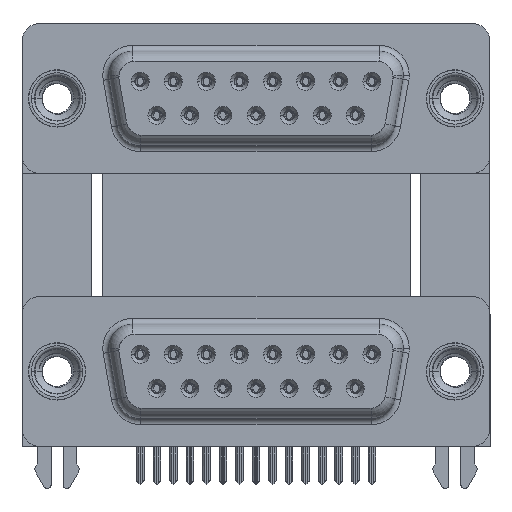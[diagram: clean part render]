
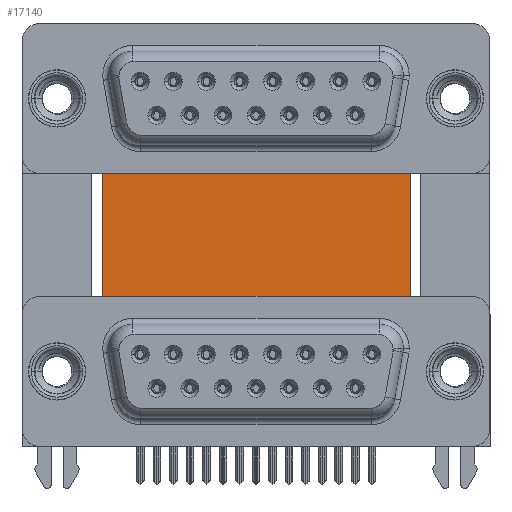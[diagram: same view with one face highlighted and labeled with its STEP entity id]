
A CAD part, top view. The second image highlights one B-rep face of the part: STEP entity #17140.
In plain terms, the highlighted planar face has unit normal (0, 0, 1).
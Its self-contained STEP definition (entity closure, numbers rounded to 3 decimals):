
#3864 = CARTESIAN_POINT ( 'NONE',  ( 3.79, 16.585, -12. ) ) ;
#4210 = EDGE_CURVE ( 'NONE', #28988, #46564, #48199, .T. ) ;
#5239 = DIRECTION ( 'NONE',  ( 0., -1., 0. ) ) ;
#5375 = PLANE ( 'NONE',  #42746 ) ;
#9090 = LINE ( 'NONE', #36530, #28786 ) ;
#13177 = CARTESIAN_POINT ( 'NONE',  ( 3.79, 16.585, -12. ) ) ;
#13573 = VECTOR ( 'NONE', #49423, 1000. ) ;
#13666 = ORIENTED_EDGE ( 'NONE', *, *, #30365, .T. ) ;
#14010 = EDGE_LOOP ( 'NONE', ( #29557, #25717, #25995, #13666 ) ) ;
#16590 = CARTESIAN_POINT ( 'NONE',  ( 29.58, 16.585, -12. ) ) ;
#16724 = EDGE_CURVE ( 'NONE', #24771, #28988, #23458, .T. ) ;
#17140 = ADVANCED_FACE ( 'NONE', ( #24380 ), #5375, .F. ) ;
#23458 = LINE ( 'NONE', #38553, #45165 ) ;
#24260 = CARTESIAN_POINT ( 'NONE',  ( 29.58, -3.735, -12. ) ) ;
#24380 = FACE_OUTER_BOUND ( 'NONE', #14010, .T. ) ;
#24771 = VERTEX_POINT ( 'NONE', #3864 ) ;
#25109 = VERTEX_POINT ( 'NONE', #41003 ) ;
#25717 = ORIENTED_EDGE ( 'NONE', *, *, #4210, .F. ) ;
#25995 = ORIENTED_EDGE ( 'NONE', *, *, #16724, .F. ) ;
#28786 = VECTOR ( 'NONE', #45262, 1000. ) ;
#28988 = VERTEX_POINT ( 'NONE', #16590 ) ;
#29557 = ORIENTED_EDGE ( 'NONE', *, *, #35198, .T. ) ;
#30365 = EDGE_CURVE ( 'NONE', #24771, #25109, #48332, .T. ) ;
#35198 = EDGE_CURVE ( 'NONE', #25109, #46564, #9090, .T. ) ;
#36530 = CARTESIAN_POINT ( 'NONE',  ( 3.79, -3.735, -12. ) ) ;
#38553 = CARTESIAN_POINT ( 'NONE',  ( 3.79, 16.585, -12. ) ) ;
#40999 = DIRECTION ( 'NONE',  ( -1., 0., 0. ) ) ;
#41003 = CARTESIAN_POINT ( 'NONE',  ( 3.79, -3.735, -12. ) ) ;
#41508 = CARTESIAN_POINT ( 'NONE',  ( 3.79, 16.585, -12. ) ) ;
#42746 = AXIS2_PLACEMENT_3D ( 'NONE', #41508, #44608, #40999 ) ;
#44076 = CARTESIAN_POINT ( 'NONE',  ( 29.58, 16.585, -12. ) ) ;
#44608 = DIRECTION ( 'NONE',  ( 0., 0., -1. ) ) ;
#45165 = VECTOR ( 'NONE', #50656, 1000. ) ;
#45262 = DIRECTION ( 'NONE',  ( 1., 0., 0. ) ) ;
#46564 = VERTEX_POINT ( 'NONE', #24260 ) ;
#47463 = VECTOR ( 'NONE', #5239, 1000. ) ;
#48199 = LINE ( 'NONE', #44076, #13573 ) ;
#48332 = LINE ( 'NONE', #13177, #47463 ) ;
#49423 = DIRECTION ( 'NONE',  ( 0., -1., 0. ) ) ;
#50656 = DIRECTION ( 'NONE',  ( 1., 0., 0. ) ) ;
